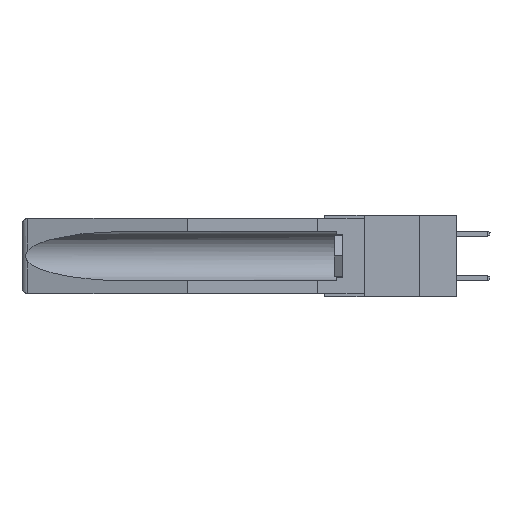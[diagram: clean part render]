
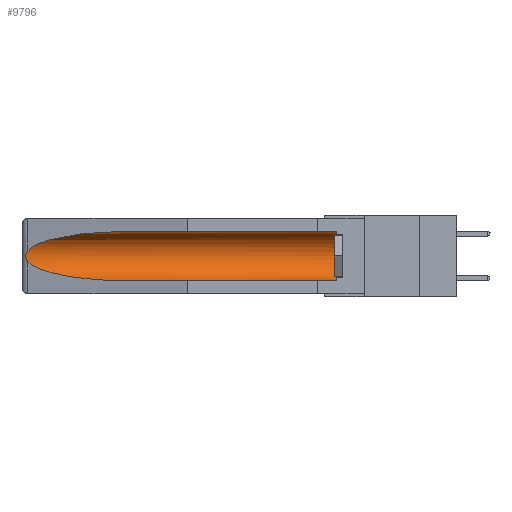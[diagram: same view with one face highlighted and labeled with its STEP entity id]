
A CAD part, left-side view. The second image highlights one B-rep face of the part: STEP entity #9796.
In plain terms, the highlighted cylindrical face has radius 2.857 mm (diameter 5.715 mm), a partial arc.
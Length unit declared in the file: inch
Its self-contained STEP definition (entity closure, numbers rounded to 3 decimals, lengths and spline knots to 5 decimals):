
#480 = FACE_OUTER_BOUND ( 'NONE', #26049, .T. ) ;
#595 = CARTESIAN_POINT ( 'NONE',  ( 0.26597, 1.5296, -0.19026 ) ) ;
#1987 = LINE ( 'NONE', #20465, #10783 ) ;
#2185 = VECTOR ( 'NONE', #18036, 39.37008 ) ;
#2829 = VERTEX_POINT ( 'NONE', #12797 ) ;
#2847 = LINE ( 'NONE', #5526, #2185 ) ;
#3904 = CARTESIAN_POINT ( 'NONE',  ( 0.155, 1.07973, -0.059 ) ) ;
#4596 = CARTESIAN_POINT ( 'NONE',  ( 0.2675, 1.53308, -0.17534 ) ) ;
#4665 = AXIS2_PLACEMENT_3D ( 'NONE', #19421, #4964, #4782 ) ;
#4782 = DIRECTION ( 'NONE',  ( 0., 0., 1. ) ) ;
#4875 = CARTESIAN_POINT ( 'NONE',  ( 0.21114, 1.30732, -0.284 ) ) ;
#4964 = DIRECTION ( 'NONE',  ( 0., -1., 0. ) ) ;
#5055 = CARTESIAN_POINT ( 'NONE',  ( 0.155, 0.126, -0.059 ) ) ;
#5373 =( BOUNDED_CURVE ( )  B_SPLINE_CURVE ( 3, ( #9164, #25670, #15302, #7344 ),
 .UNSPECIFIED., .F., .F. ) 
 B_SPLINE_CURVE_WITH_KNOTS ( ( 4, 4 ),
 ( 4.71239, 6.08839 ),
 .UNSPECIFIED. ) 
 CURVE ( )  GEOMETRIC_REPRESENTATION_ITEM ( )  RATIONAL_B_SPLINE_CURVE ( ( 1., 0.848, 0.848, 1. ) ) 
 REPRESENTATION_ITEM ( '' )  );
#5414 = VERTEX_POINT ( 'NONE', #5055 ) ;
#5526 = CARTESIAN_POINT ( 'NONE',  ( 0.155, -0.30754, -0.284 ) ) ;
#6757 = CARTESIAN_POINT ( 'NONE',  ( 0.26597, 1.52961, -0.15275 ) ) ;
#6948 = CARTESIAN_POINT ( 'NONE',  ( 0.155, 1.07973, -0.284 ) ) ;
#7344 = CARTESIAN_POINT ( 'NONE',  ( 0.26537, 1.52718, -0.14972 ) ) ;
#7775 = EDGE_CURVE ( 'NONE', #11217, #2829, #2847, .T. ) ;
#8322 = ORIENTED_EDGE ( 'NONE', *, *, #12456, .T. ) ;
#9060 = CARTESIAN_POINT ( 'NONE',  ( 0.2673, 1.5327, -0.16383 ) ) ;
#9164 = CARTESIAN_POINT ( 'NONE',  ( 0.155, 1.07973, -0.059 ) ) ;
#9796 = ADVANCED_FACE ( 'NONE', ( #480 ), #19248, .F. ) ;
#10218 = DIRECTION ( 'NONE',  ( 0., 1., 0. ) ) ;
#10259 = CARTESIAN_POINT ( 'NONE',  ( 0.155, -0.30754, -0.1715 ) ) ;
#10783 = VECTOR ( 'NONE', #10218, 39.37008 ) ;
#10951 = CARTESIAN_POINT ( 'NONE',  ( 0.2675, 1.53308, -0.16763 ) ) ;
#11217 = VERTEX_POINT ( 'NONE', #25245 ) ;
#11976 = ORIENTED_EDGE ( 'NONE', *, *, #14598, .T. ) ;
#12247 = ORIENTED_EDGE ( 'NONE', *, *, #18449, .T. ) ;
#12456 = EDGE_CURVE ( 'NONE', #16171, #19195, #17008, .T. ) ;
#12797 = CARTESIAN_POINT ( 'NONE',  ( 0.155, 1.07973, -0.284 ) ) ;
#13857 =( BOUNDED_CURVE ( )  B_SPLINE_CURVE ( 3, ( #21473, #25288, #4875, #6948 ),
 .UNSPECIFIED., .F., .F. ) 
 B_SPLINE_CURVE_WITH_KNOTS ( ( 4, 4 ),
 ( 0.1948, 1.5708 ),
 .UNSPECIFIED. ) 
 CURVE ( )  GEOMETRIC_REPRESENTATION_ITEM ( )  RATIONAL_B_SPLINE_CURVE ( ( 1., 0.848, 0.848, 1. ) ) 
 REPRESENTATION_ITEM ( '' )  );
#14562 = EDGE_CURVE ( 'NONE', #19195, #2829, #13857, .T. ) ;
#14598 = EDGE_CURVE ( 'NONE', #11217, #5414, #16092, .T. ) ;
#14925 = CARTESIAN_POINT ( 'NONE',  ( 0.26537, 1.52718, -0.19328 ) ) ;
#15104 = CARTESIAN_POINT ( 'NONE',  ( 0.2673, 1.53269, -0.17917 ) ) ;
#15302 = CARTESIAN_POINT ( 'NONE',  ( 0.25451, 1.48313, -0.09465 ) ) ;
#16092 = CIRCLE ( 'NONE', #4665, 0.1125 ) ;
#16171 = VERTEX_POINT ( 'NONE', #18859 ) ;
#16928 = ORIENTED_EDGE ( 'NONE', *, *, #7775, .F. ) ;
#17008 = B_SPLINE_CURVE_WITH_KNOTS ( 'NONE', 3,
 ( #17118, #6757, #19143, #9060, #10951, #4596, #15104, #25570, #595, #25376 ),
 .UNSPECIFIED., .F., .F.,
 ( 4, 2, 2, 2, 4 ),
 ( 0., 0.00029, 0.00058, 0.00087, 0.00117 ),
 .UNSPECIFIED. ) ;
#17118 = CARTESIAN_POINT ( 'NONE',  ( 0.26537, 1.52718, -0.14972 ) ) ;
#18036 = DIRECTION ( 'NONE',  ( 0., 1., 0. ) ) ;
#18449 = EDGE_CURVE ( 'NONE', #26423, #16171, #5373, .T. ) ;
#18859 = CARTESIAN_POINT ( 'NONE',  ( 0.26537, 1.52718, -0.14972 ) ) ;
#19143 = CARTESIAN_POINT ( 'NONE',  ( 0.26654, 1.53092, -0.15636 ) ) ;
#19195 = VERTEX_POINT ( 'NONE', #14925 ) ;
#19248 = CYLINDRICAL_SURFACE ( 'NONE', #24310, 0.1125 ) ;
#19421 = CARTESIAN_POINT ( 'NONE',  ( 0.155, 0.126, -0.1715 ) ) ;
#20457 = ORIENTED_EDGE ( 'NONE', *, *, #24678, .T. ) ;
#20465 = CARTESIAN_POINT ( 'NONE',  ( 0.155, -0.30754, -0.059 ) ) ;
#20771 = DIRECTION ( 'NONE',  ( 0., 1., 0. ) ) ;
#20984 = ORIENTED_EDGE ( 'NONE', *, *, #14562, .T. ) ;
#21473 = CARTESIAN_POINT ( 'NONE',  ( 0.26537, 1.52718, -0.19328 ) ) ;
#24310 = AXIS2_PLACEMENT_3D ( 'NONE', #10259, #20771, #25406 ) ;
#24678 = EDGE_CURVE ( 'NONE', #5414, #26423, #1987, .T. ) ;
#25245 = CARTESIAN_POINT ( 'NONE',  ( 0.155, 0.126, -0.284 ) ) ;
#25288 = CARTESIAN_POINT ( 'NONE',  ( 0.25451, 1.48313, -0.24835 ) ) ;
#25376 = CARTESIAN_POINT ( 'NONE',  ( 0.26537, 1.52718, -0.19328 ) ) ;
#25406 = DIRECTION ( 'NONE',  ( 0., 0., 1. ) ) ;
#25570 = CARTESIAN_POINT ( 'NONE',  ( 0.26655, 1.53094, -0.18657 ) ) ;
#25670 = CARTESIAN_POINT ( 'NONE',  ( 0.21114, 1.30732, -0.059 ) ) ;
#26049 = EDGE_LOOP ( 'NONE', ( #12247, #8322, #20984, #16928, #11976, #20457 ) ) ;
#26423 = VERTEX_POINT ( 'NONE', #3904 ) ;
